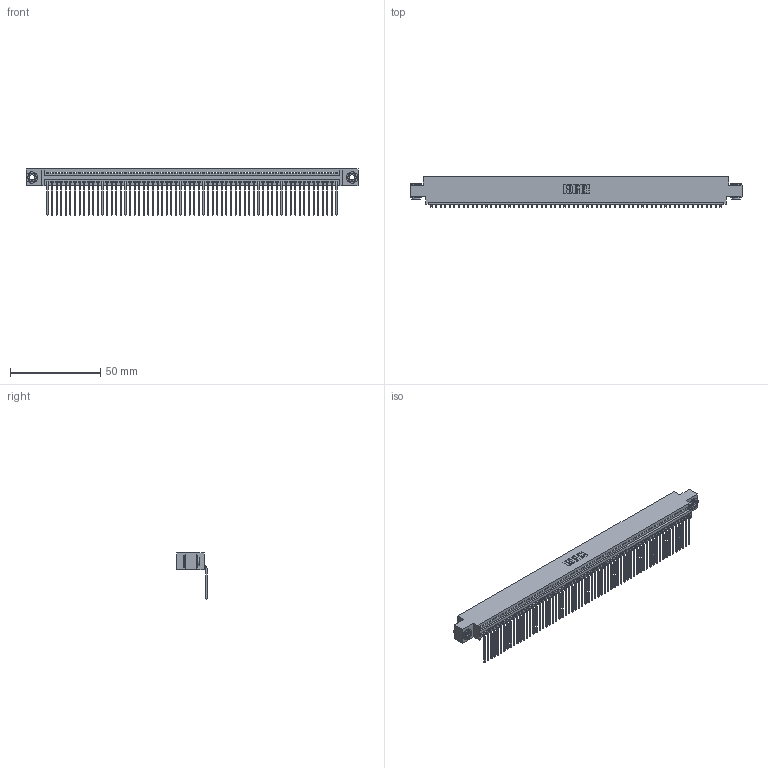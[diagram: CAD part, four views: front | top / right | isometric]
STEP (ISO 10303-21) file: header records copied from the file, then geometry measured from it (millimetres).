
FILE_DESCRIPTION (( 'STEP AP203' ), '1' );
FILE_NAME ('395-064-559-603.STEP', '2019-10-25T03:42:50', ( '' ), ( '' ), 'SwSTEP 2.0', 'SolidWorks 2016', '' );
FILE_SCHEMA (( 'CONFIG_CONTROL_DESIGN' ));
Length unit declared in the file: inch
Products named in the file (4): 345-250-002_345-250-002-102; 395-064-559-603; 345 Part_0.170 Offset - 0.156 Dia-TH; 345-292-001_558 559 Tail - 1
Assembly tree (67 placements, depth 2):
  395-064-559-603
    345 Part_0.170 Offset - 0.156 Dia-TH
    345-292-001_558 559 Tail - 1  x64
    345-250-002_345-250-002-102  x2
Bounding box: 183.77 x 16.75 x 25.53 mm (x, y, z)
Volume: 17754 mm3; surface area: 25486.5 mm2
Topology: 67 solids, 67 shells, 4008 faces, 12077 edges, 7962 vertices
Faces by surface type: plane 2782, cylinder 1218, cone 8
Entity records: 46072 total; most frequent: CARTESIAN_POINT 7959, ORIENTED_EDGE 7950, DIRECTION 6949, EDGE_CURVE 3975, VECTOR 3563, LINE 3563, VERTEX_POINT 2646, AXIS2_PLACEMENT_3D 1693
